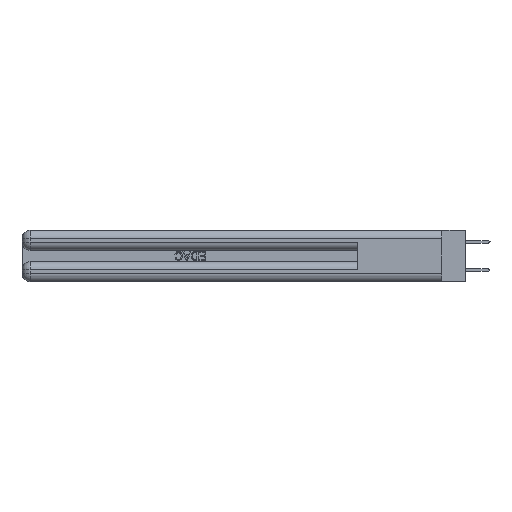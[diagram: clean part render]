
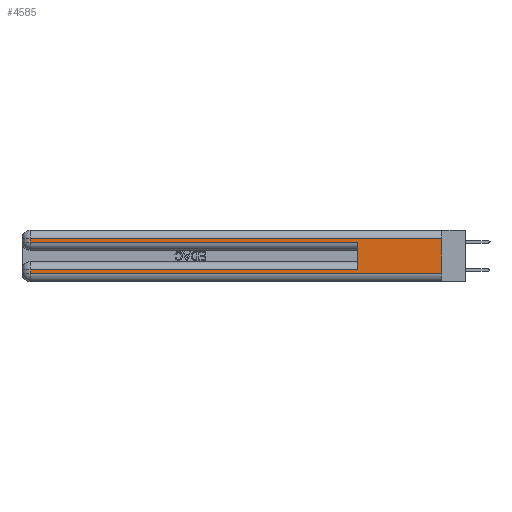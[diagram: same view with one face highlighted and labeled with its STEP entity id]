
A CAD part, left-side view. The second image highlights one B-rep face of the part: STEP entity #4585.
In plain terms, the highlighted planar face has unit normal (-1, 0, 0).
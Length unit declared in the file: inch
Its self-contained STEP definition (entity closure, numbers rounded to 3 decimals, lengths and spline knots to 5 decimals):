
#1966 = EDGE_LOOP ( 'NONE', ( #38205, #24121, #2268, #24462, #37044, #27183, #33435, #33039 ) ) ;
#2268 = ORIENTED_EDGE ( 'NONE', *, *, #17465, .T. ) ;
#2274 = DIRECTION ( 'NONE',  ( 0., 0., 1. ) ) ;
#4216 = LINE ( 'NONE', #11563, #35300 ) ;
#4243 = CARTESIAN_POINT ( 'NONE',  ( 0., 2.94, 0.085 ) ) ;
#4442 = CARTESIAN_POINT ( 'NONE',  ( 0., 0., 0.31 ) ) ;
#4585 = ADVANCED_FACE ( 'NONE', ( #18681 ), #28213, .F. ) ;
#4756 = CARTESIAN_POINT ( 'NONE',  ( 0., 0., 0.37 ) ) ;
#5023 = DIRECTION ( 'NONE',  ( 0., 0., -1. ) ) ;
#7927 = VECTOR ( 'NONE', #5023, 39.37008 ) ;
#8665 = LINE ( 'NONE', #18273, #35540 ) ;
#10098 = DIRECTION ( 'NONE',  ( 0., -1., 0. ) ) ;
#10567 = CARTESIAN_POINT ( 'NONE',  ( 0., 0.6, 0.285 ) ) ;
#10894 = VECTOR ( 'NONE', #2274, 39.37008 ) ;
#10931 = CARTESIAN_POINT ( 'NONE',  ( 0., 0.6, 0.145 ) ) ;
#11020 = VERTEX_POINT ( 'NONE', #25362 ) ;
#11563 = CARTESIAN_POINT ( 'NONE',  ( 0., 0., 0.285 ) ) ;
#12059 = CARTESIAN_POINT ( 'NONE',  ( 0., 2.94, 0.06 ) ) ;
#12121 = VECTOR ( 'NONE', #12222, 39.37008 ) ;
#12222 = DIRECTION ( 'NONE',  ( 0., -1., 0. ) ) ;
#12430 = LINE ( 'NONE', #24569, #33617 ) ;
#12669 = VERTEX_POINT ( 'NONE', #13464 ) ;
#13464 = CARTESIAN_POINT ( 'NONE',  ( 0., 0.6, 0.085 ) ) ;
#14196 = LINE ( 'NONE', #10931, #10894 ) ;
#14384 = LINE ( 'NONE', #23876, #37465 ) ;
#15087 = CARTESIAN_POINT ( 'NONE',  ( 0., 0., 0.06 ) ) ;
#16007 = AXIS2_PLACEMENT_3D ( 'NONE', #25455, #28948, #31955 ) ;
#16385 = EDGE_CURVE ( 'NONE', #36867, #16925, #37537, .T. ) ;
#16925 = VERTEX_POINT ( 'NONE', #15087 ) ;
#17465 = EDGE_CURVE ( 'NONE', #24928, #19173, #14384, .T. ) ;
#17502 = CARTESIAN_POINT ( 'NONE',  ( 0., 2.94, 0.285 ) ) ;
#18273 = CARTESIAN_POINT ( 'NONE',  ( 0., 0., 0.085 ) ) ;
#18681 = FACE_OUTER_BOUND ( 'NONE', #1966, .T. ) ;
#19173 = VERTEX_POINT ( 'NONE', #17502 ) ;
#19767 = CARTESIAN_POINT ( 'NONE',  ( 0., 2.94, 0.31 ) ) ;
#20179 = EDGE_CURVE ( 'NONE', #12669, #36029, #14196, .T. ) ;
#21164 = DIRECTION ( 'NONE',  ( 0., 0., -1. ) ) ;
#22350 = LINE ( 'NONE', #4442, #27997 ) ;
#23876 = CARTESIAN_POINT ( 'NONE',  ( 0., 2.94, 0.37 ) ) ;
#24121 = ORIENTED_EDGE ( 'NONE', *, *, #32923, .T. ) ;
#24462 = ORIENTED_EDGE ( 'NONE', *, *, #30797, .T. ) ;
#24569 = CARTESIAN_POINT ( 'NONE',  ( 0., 2.94, 0.37 ) ) ;
#24928 = VERTEX_POINT ( 'NONE', #19767 ) ;
#25362 = CARTESIAN_POINT ( 'NONE',  ( 0., 0., 0.31 ) ) ;
#25455 = CARTESIAN_POINT ( 'NONE',  ( 0., 0., 0.37 ) ) ;
#27183 = ORIENTED_EDGE ( 'NONE', *, *, #33707, .T. ) ;
#27997 = VECTOR ( 'NONE', #31132, 39.37008 ) ;
#28213 = PLANE ( 'NONE',  #16007 ) ;
#28650 = LINE ( 'NONE', #4756, #7927 ) ;
#28948 = DIRECTION ( 'NONE',  ( 1., 0., 0. ) ) ;
#29772 = DIRECTION ( 'NONE',  ( 0., 0., -1. ) ) ;
#30085 = DIRECTION ( 'NONE',  ( 0., 1., 0. ) ) ;
#30498 = CARTESIAN_POINT ( 'NONE',  ( 0., 0., 0.06 ) ) ;
#30797 = EDGE_CURVE ( 'NONE', #19173, #36029, #4216, .T. ) ;
#31132 = DIRECTION ( 'NONE',  ( 0., 1., 0. ) ) ;
#31955 = DIRECTION ( 'NONE',  ( 0., 0., -1. ) ) ;
#32923 = EDGE_CURVE ( 'NONE', #11020, #24928, #22350, .T. ) ;
#33039 = ORIENTED_EDGE ( 'NONE', *, *, #16385, .T. ) ;
#33435 = ORIENTED_EDGE ( 'NONE', *, *, #33593, .T. ) ;
#33593 = EDGE_CURVE ( 'NONE', #37961, #36867, #12430, .T. ) ;
#33617 = VECTOR ( 'NONE', #21164, 39.37008 ) ;
#33707 = EDGE_CURVE ( 'NONE', #12669, #37961, #8665, .T. ) ;
#34677 = EDGE_CURVE ( 'NONE', #11020, #16925, #28650, .T. ) ;
#35300 = VECTOR ( 'NONE', #10098, 39.37008 ) ;
#35540 = VECTOR ( 'NONE', #30085, 39.37008 ) ;
#36029 = VERTEX_POINT ( 'NONE', #10567 ) ;
#36867 = VERTEX_POINT ( 'NONE', #12059 ) ;
#37044 = ORIENTED_EDGE ( 'NONE', *, *, #20179, .F. ) ;
#37465 = VECTOR ( 'NONE', #29772, 39.37008 ) ;
#37537 = LINE ( 'NONE', #30498, #12121 ) ;
#37961 = VERTEX_POINT ( 'NONE', #4243 ) ;
#38205 = ORIENTED_EDGE ( 'NONE', *, *, #34677, .F. ) ;
